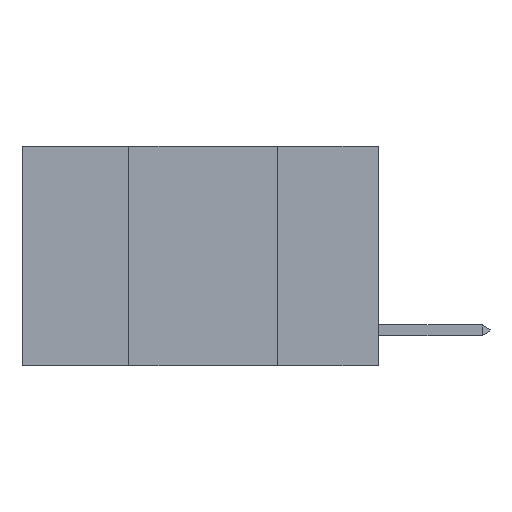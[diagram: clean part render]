
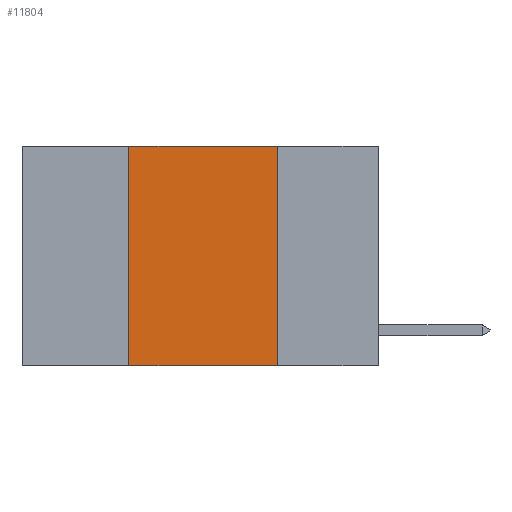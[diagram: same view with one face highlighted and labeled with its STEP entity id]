
A CAD part, left-side view. The second image highlights one B-rep face of the part: STEP entity #11804.
In plain terms, the highlighted planar face has unit normal (-1, 0, 0).
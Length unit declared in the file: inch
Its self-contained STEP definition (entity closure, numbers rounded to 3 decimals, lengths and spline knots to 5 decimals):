
#34 = ORIENTED_EDGE ( 'NONE', *, *, #3262, .T. ) ;
#496 = DIRECTION ( 'NONE',  ( 0., 0., -1. ) ) ;
#1174 = VECTOR ( 'NONE', #6074, 39.37008 ) ;
#1660 = VECTOR ( 'NONE', #7053, 39.37008 ) ;
#1782 = CARTESIAN_POINT ( 'NONE',  ( 0., 0.42, 0. ) ) ;
#2262 = CARTESIAN_POINT ( 'NONE',  ( 0., 0.6, -0.37 ) ) ;
#3262 = EDGE_CURVE ( 'NONE', #11556, #7129, #10371, .T. ) ;
#3330 = EDGE_CURVE ( 'NONE', #7594, #13098, #12314, .T. ) ;
#3658 = FACE_OUTER_BOUND ( 'NONE', #12719, .T. ) ;
#4318 = PLANE ( 'NONE',  #14387 ) ;
#4467 = ORIENTED_EDGE ( 'NONE', *, *, #11475, .F. ) ;
#5310 = DIRECTION ( 'NONE',  ( 1., 0., 0. ) ) ;
#5353 = CARTESIAN_POINT ( 'NONE',  ( 0., 0.42, 0. ) ) ;
#5412 = CARTESIAN_POINT ( 'NONE',  ( 0., 0.42, -0.37 ) ) ;
#6074 = DIRECTION ( 'NONE',  ( 0., -1., 0. ) ) ;
#7053 = DIRECTION ( 'NONE',  ( 0., 0., 1. ) ) ;
#7129 = VERTEX_POINT ( 'NONE', #10363 ) ;
#7594 = VERTEX_POINT ( 'NONE', #5353 ) ;
#8272 = DIRECTION ( 'NONE',  ( 0., 0., -1. ) ) ;
#9573 = DIRECTION ( 'NONE',  ( 0., -1., 0. ) ) ;
#10363 = CARTESIAN_POINT ( 'NONE',  ( 0., 0.17, -0.37 ) ) ;
#10371 = LINE ( 'NONE', #2262, #12306 ) ;
#11456 = LINE ( 'NONE', #1782, #1660 ) ;
#11475 = EDGE_CURVE ( 'NONE', #13098, #7129, #11971, .T. ) ;
#11556 = VERTEX_POINT ( 'NONE', #5412 ) ;
#11804 = ADVANCED_FACE ( 'NONE', ( #3658 ), #4318, .F. ) ;
#11971 = LINE ( 'NONE', #13079, #15400 ) ;
#12306 = VECTOR ( 'NONE', #9573, 39.37008 ) ;
#12314 = LINE ( 'NONE', #14633, #1174 ) ;
#12719 = EDGE_LOOP ( 'NONE', ( #4467, #13075, #14038, #34 ) ) ;
#13075 = ORIENTED_EDGE ( 'NONE', *, *, #3330, .F. ) ;
#13079 = CARTESIAN_POINT ( 'NONE',  ( 0., 0.17, 0. ) ) ;
#13098 = VERTEX_POINT ( 'NONE', #15457 ) ;
#14038 = ORIENTED_EDGE ( 'NONE', *, *, #15281, .F. ) ;
#14387 = AXIS2_PLACEMENT_3D ( 'NONE', #15408, #5310, #496 ) ;
#14633 = CARTESIAN_POINT ( 'NONE',  ( 0., 0.6, 0. ) ) ;
#15281 = EDGE_CURVE ( 'NONE', #11556, #7594, #11456, .T. ) ;
#15400 = VECTOR ( 'NONE', #8272, 39.37008 ) ;
#15408 = CARTESIAN_POINT ( 'NONE',  ( 0., 0.6, 0. ) ) ;
#15457 = CARTESIAN_POINT ( 'NONE',  ( 0., 0.17, 0. ) ) ;
